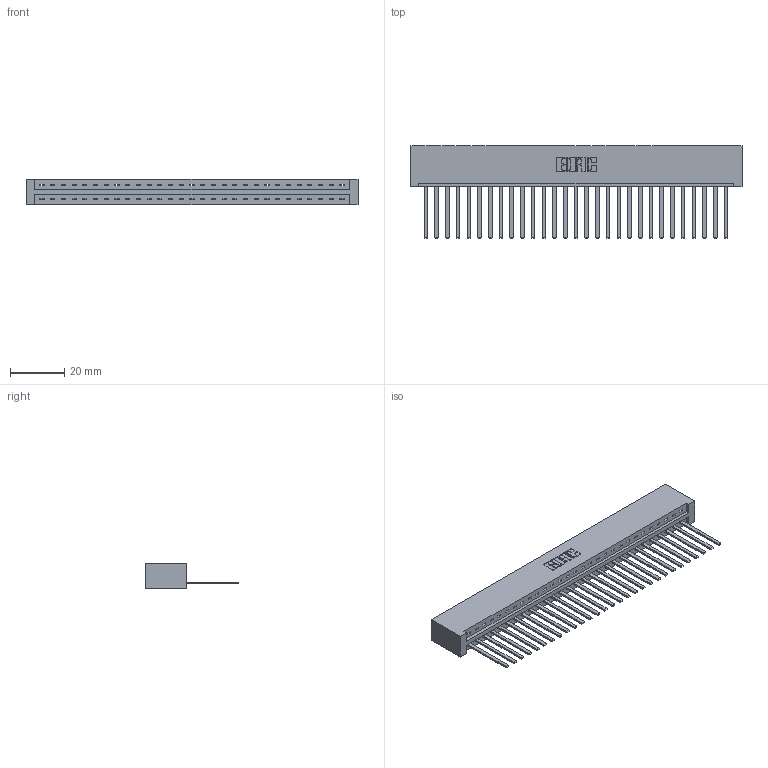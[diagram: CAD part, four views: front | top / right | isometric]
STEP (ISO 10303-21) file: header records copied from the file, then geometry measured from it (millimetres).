
FILE_DESCRIPTION (( 'STEP AP203' ), '1' );
FILE_NAME ('387-029-544-101.STEP', '2019-10-03T17:27:14', ( '' ), ( '' ), 'SwSTEP 2.0', 'SolidWorks 2016', '' );
FILE_SCHEMA (( 'CONFIG_CONTROL_DESIGN' ));
Length unit declared in the file: inch
Products named in the file (3): 387-029-544-101; 345-292-001_345-293-144; 337 Part_No Mounting Lugs
Assembly tree (30 placements, depth 2):
  387-029-544-101
    337 Part_No Mounting Lugs
    345-292-001_345-293-144  x29
Bounding box: 122.78 x 34.3 x 9.4 mm (x, y, z)
Volume: 13673.2 mm3; surface area: 15143.3 mm2
Topology: 30 solids, 30 shells, 1730 faces, 5217 edges, 3438 vertices
Faces by surface type: plane 1284, cylinder 446
Entity records: 22777 total; most frequent: CARTESIAN_POINT 3973, ORIENTED_EDGE 3938, DIRECTION 3359, EDGE_CURVE 1969, LINE 1853, VECTOR 1853, VERTEX_POINT 1310, AXIS2_PLACEMENT_3D 753
